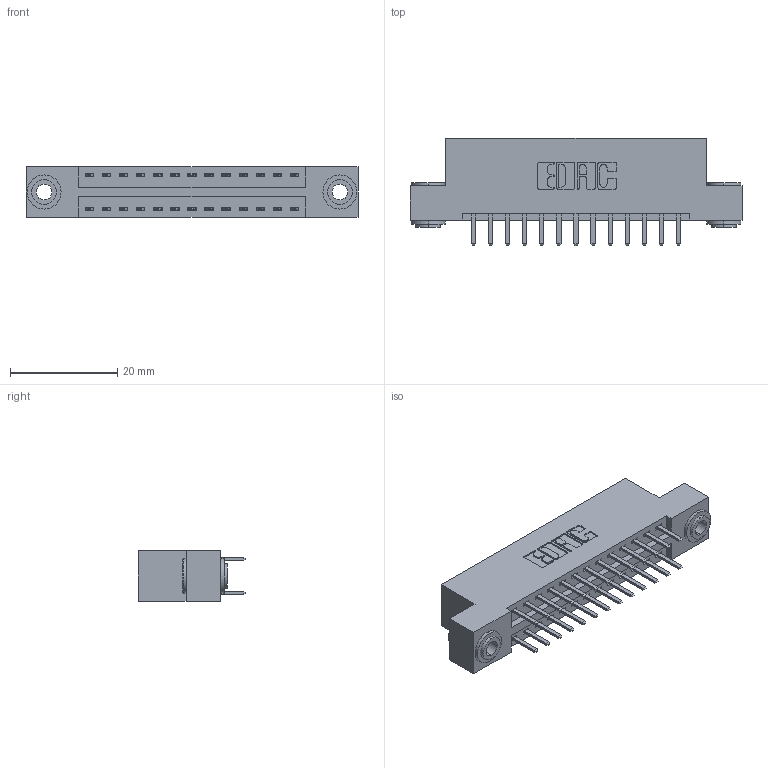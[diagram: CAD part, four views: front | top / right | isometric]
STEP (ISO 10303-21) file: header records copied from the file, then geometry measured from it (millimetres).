
FILE_DESCRIPTION (( 'STEP AP203' ), '1' );
FILE_NAME ('396-026-520-203.STEP', '2018-09-04T23:13:50', ( '' ), ( '' ), 'SwSTEP 2.0', 'SolidWorks 2016', '' );
FILE_SCHEMA (( 'CONFIG_CONTROL_DESIGN' ));
Length unit declared in the file: inch
Products named in the file (4): 346 Part_Flush Mounting Lugs - 0.156 Dia-TH; 345-292-001_345-293-120; 345-250-002_345-250-002-102; 396-026-520-203
Assembly tree (29 placements, depth 2):
  396-026-520-203
    346 Part_Flush Mounting Lugs - 0.156 Dia-TH
    345-292-001_345-293-120  x26
    345-250-002_345-250-002-102  x2
Bounding box: 61.85 x 20.02 x 9.4 mm (x, y, z)
Volume: 5813.8 mm3; surface area: 7723 mm2
Topology: 29 solids, 29 shells, 1616 faces, 4643 edges, 3022 vertices
Faces by surface type: plane 1048, cylinder 560, cone 8
Entity records: 13152 total; most frequent: CARTESIAN_POINT 2195, ORIENTED_EDGE 2110, DIRECTION 2005, EDGE_CURVE 1055, VECTOR 843, LINE 843, VERTEX_POINT 698, AXIS2_PLACEMENT_3D 581
